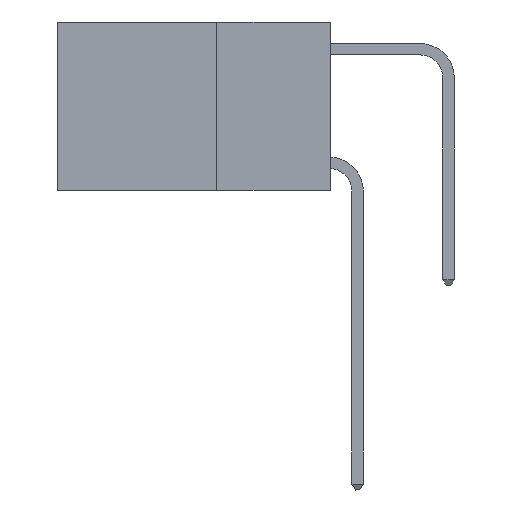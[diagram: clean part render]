
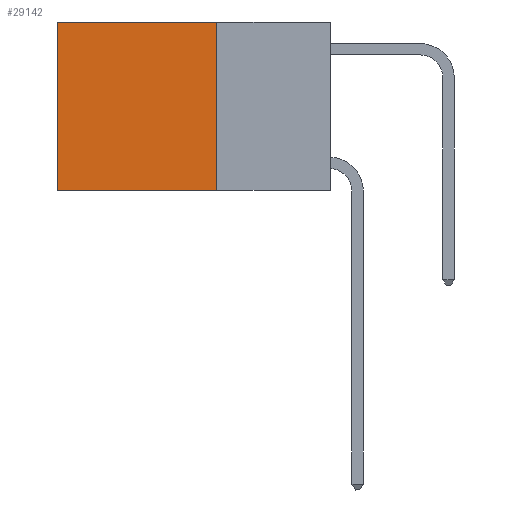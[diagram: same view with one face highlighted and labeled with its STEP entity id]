
A CAD part, left-side view. The second image highlights one B-rep face of the part: STEP entity #29142.
In plain terms, the highlighted planar face has unit normal (-1, 0, 0).
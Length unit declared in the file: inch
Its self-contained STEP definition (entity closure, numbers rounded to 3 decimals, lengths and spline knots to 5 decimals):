
#2075 = DIRECTION ( 'NONE',  ( 0., 1., 0. ) ) ;
#2654 = FACE_OUTER_BOUND ( 'NONE', #4133, .T. ) ;
#2895 = CARTESIAN_POINT ( 'NONE',  ( 0.2625, 0.25, 0. ) ) ;
#3697 = LINE ( 'NONE', #2895, #27057 ) ;
#3883 = LINE ( 'NONE', #4372, #15218 ) ;
#4133 = EDGE_LOOP ( 'NONE', ( #26864, #20017, #19348, #18920 ) ) ;
#4372 = CARTESIAN_POINT ( 'NONE',  ( 0.2625, 0.25, 0. ) ) ;
#5150 = LINE ( 'NONE', #17940, #16467 ) ;
#6245 = LINE ( 'NONE', #15451, #23608 ) ;
#6289 = VERTEX_POINT ( 'NONE', #17321 ) ;
#6531 = VERTEX_POINT ( 'NONE', #13553 ) ;
#7189 = VERTEX_POINT ( 'NONE', #27372 ) ;
#7810 = VERTEX_POINT ( 'NONE', #20423 ) ;
#8751 = DIRECTION ( 'NONE',  ( 0., 1., 0. ) ) ;
#9451 = CARTESIAN_POINT ( 'NONE',  ( 0.2625, 0.25, 0. ) ) ;
#11756 = DIRECTION ( 'NONE',  ( 1., 0., 0. ) ) ;
#13553 = CARTESIAN_POINT ( 'NONE',  ( 0.2625, 0.25, 0. ) ) ;
#15218 = VECTOR ( 'NONE', #2075, 39.37008 ) ;
#15451 = CARTESIAN_POINT ( 'NONE',  ( 0.2625, 0.25, -0.37 ) ) ;
#16467 = VECTOR ( 'NONE', #20214, 39.37008 ) ;
#16682 = EDGE_CURVE ( 'NONE', #6531, #7810, #3697, .T. ) ;
#17321 = CARTESIAN_POINT ( 'NONE',  ( 0.2625, 0.6, -0.37 ) ) ;
#17940 = CARTESIAN_POINT ( 'NONE',  ( 0.2625, 0.6, 0. ) ) ;
#18920 = ORIENTED_EDGE ( 'NONE', *, *, #21749, .T. ) ;
#19348 = ORIENTED_EDGE ( 'NONE', *, *, #16682, .F. ) ;
#19550 = AXIS2_PLACEMENT_3D ( 'NONE', #9451, #11756, #27572 ) ;
#20017 = ORIENTED_EDGE ( 'NONE', *, *, #20859, .F. ) ;
#20214 = DIRECTION ( 'NONE',  ( 0., 0., -1. ) ) ;
#20423 = CARTESIAN_POINT ( 'NONE',  ( 0.2625, 0.25, -0.37 ) ) ;
#20859 = EDGE_CURVE ( 'NONE', #7810, #6289, #6245, .T. ) ;
#21749 = EDGE_CURVE ( 'NONE', #6531, #7189, #3883, .T. ) ;
#22998 = PLANE ( 'NONE',  #19550 ) ;
#23608 = VECTOR ( 'NONE', #8751, 39.37008 ) ;
#24392 = EDGE_CURVE ( 'NONE', #7189, #6289, #5150, .T. ) ;
#25463 = DIRECTION ( 'NONE',  ( 0., 0., -1. ) ) ;
#26864 = ORIENTED_EDGE ( 'NONE', *, *, #24392, .T. ) ;
#27057 = VECTOR ( 'NONE', #25463, 39.37008 ) ;
#27372 = CARTESIAN_POINT ( 'NONE',  ( 0.2625, 0.6, 0. ) ) ;
#27572 = DIRECTION ( 'NONE',  ( 0., 0., -1. ) ) ;
#29142 = ADVANCED_FACE ( 'NONE', ( #2654 ), #22998, .F. ) ;
